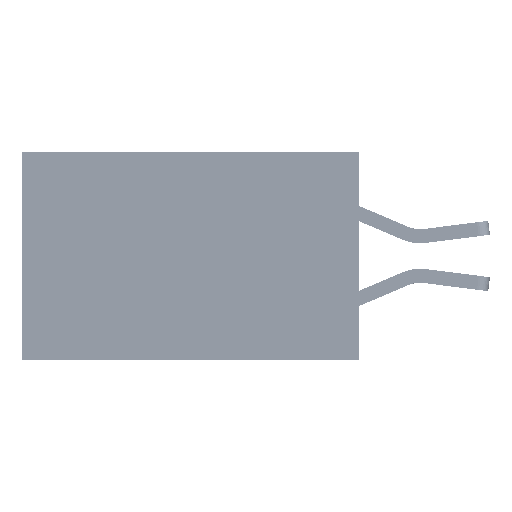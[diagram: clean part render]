
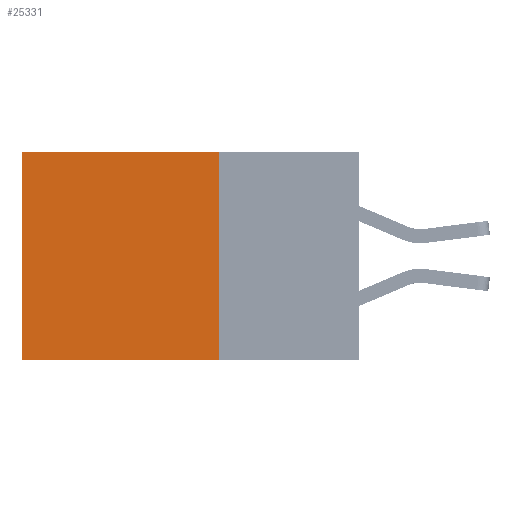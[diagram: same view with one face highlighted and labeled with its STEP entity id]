
A CAD part, left-side view. The second image highlights one B-rep face of the part: STEP entity #25331.
In plain terms, the highlighted planar face has unit normal (-1, 0, 0).
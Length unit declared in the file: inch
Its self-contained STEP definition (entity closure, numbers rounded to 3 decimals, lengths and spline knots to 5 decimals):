
#638 = EDGE_CURVE ( 'NONE', #44653, #24879, #37676, .T. ) ;
#791 = CARTESIAN_POINT ( 'NONE',  ( 0.2875, 0.25, 0. ) ) ;
#2724 = EDGE_CURVE ( 'NONE', #41774, #23434, #22473, .T. ) ;
#4218 = DIRECTION ( 'NONE',  ( 0., 0., -1. ) ) ;
#4568 = DIRECTION ( 'NONE',  ( 0., 0., -1. ) ) ;
#5092 = CARTESIAN_POINT ( 'NONE',  ( 0.2875, 0.25, -0.37 ) ) ;
#9155 = ORIENTED_EDGE ( 'NONE', *, *, #24876, .T. ) ;
#9206 = VECTOR ( 'NONE', #27542, 39.37008 ) ;
#10271 = CARTESIAN_POINT ( 'NONE',  ( 0.2875, 0.25, -0.37 ) ) ;
#12515 = ORIENTED_EDGE ( 'NONE', *, *, #27283, .F. ) ;
#12857 = VECTOR ( 'NONE', #41291, 39.37008 ) ;
#15935 = DIRECTION ( 'NONE',  ( 1., 0., 0. ) ) ;
#16692 = CARTESIAN_POINT ( 'NONE',  ( 0.2875, 0.6, 0. ) ) ;
#17393 = LINE ( 'NONE', #10271, #9206 ) ;
#18141 = CARTESIAN_POINT ( 'NONE',  ( 0.2875, 0.6, -0.37 ) ) ;
#20655 = CARTESIAN_POINT ( 'NONE',  ( 0.2875, 0.25, 0. ) ) ;
#22473 = LINE ( 'NONE', #25777, #39127 ) ;
#23322 = LINE ( 'NONE', #30415, #12857 ) ;
#23434 = VERTEX_POINT ( 'NONE', #18141 ) ;
#24876 = EDGE_CURVE ( 'NONE', #44653, #41774, #23322, .T. ) ;
#24879 = VERTEX_POINT ( 'NONE', #5092 ) ;
#25331 = ADVANCED_FACE ( 'NONE', ( #26580 ), #33674, .F. ) ;
#25777 = CARTESIAN_POINT ( 'NONE',  ( 0.2875, 0.6, 0. ) ) ;
#25877 = ORIENTED_EDGE ( 'NONE', *, *, #2724, .T. ) ;
#26580 = FACE_OUTER_BOUND ( 'NONE', #32094, .T. ) ;
#26996 = CARTESIAN_POINT ( 'NONE',  ( 0.2875, 0.25, 0. ) ) ;
#27283 = EDGE_CURVE ( 'NONE', #24879, #23434, #17393, .T. ) ;
#27542 = DIRECTION ( 'NONE',  ( 0., 1., 0. ) ) ;
#30415 = CARTESIAN_POINT ( 'NONE',  ( 0.2875, 0.25, 0. ) ) ;
#32094 = EDGE_LOOP ( 'NONE', ( #25877, #12515, #37329, #9155 ) ) ;
#33674 = PLANE ( 'NONE',  #34030 ) ;
#34030 = AXIS2_PLACEMENT_3D ( 'NONE', #791, #15935, #4568 ) ;
#37329 = ORIENTED_EDGE ( 'NONE', *, *, #638, .F. ) ;
#37676 = LINE ( 'NONE', #20655, #43365 ) ;
#39127 = VECTOR ( 'NONE', #4218, 39.37008 ) ;
#41291 = DIRECTION ( 'NONE',  ( 0., 1., 0. ) ) ;
#41774 = VERTEX_POINT ( 'NONE', #16692 ) ;
#43365 = VECTOR ( 'NONE', #45716, 39.37008 ) ;
#44653 = VERTEX_POINT ( 'NONE', #26996 ) ;
#45716 = DIRECTION ( 'NONE',  ( 0., 0., -1. ) ) ;
